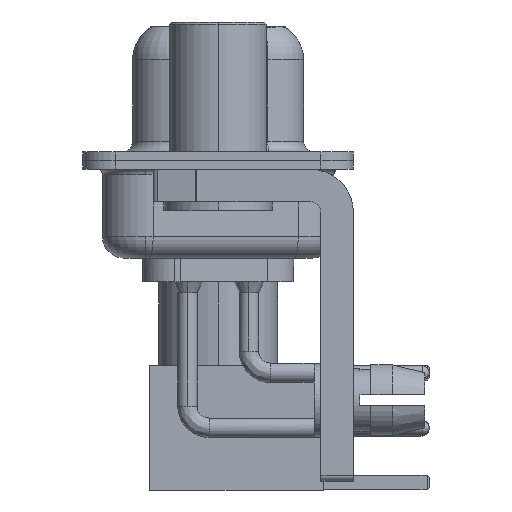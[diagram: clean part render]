
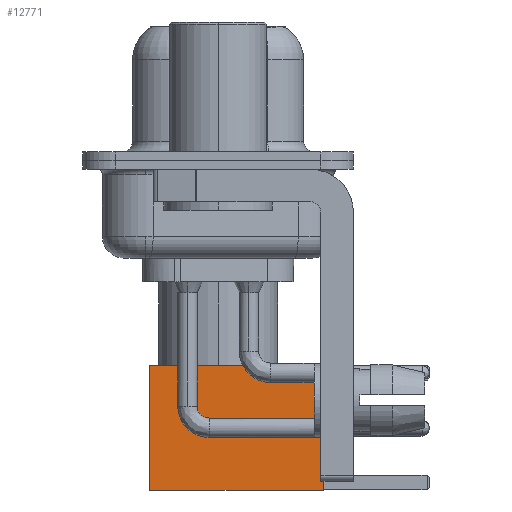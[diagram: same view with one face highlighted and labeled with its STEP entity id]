
A CAD part, left-side view. The second image highlights one B-rep face of the part: STEP entity #12771.
In plain terms, the highlighted face is planar.
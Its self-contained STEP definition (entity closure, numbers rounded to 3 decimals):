
#80 = FACE_OUTER_BOUND ( 'NONE', #11732, .T. ) ;
#1026 = LINE ( 'NONE', #19393, #6823 ) ;
#2244 = DIRECTION ( 'NONE',  ( 0., 0., -1. ) ) ;
#2800 = CARTESIAN_POINT ( 'NONE',  ( 2.875, 2.875, 8. ) ) ;
#3455 = ORIENTED_EDGE ( 'NONE', *, *, #25494, .T. ) ;
#4696 = DIRECTION ( 'NONE',  ( 0., 0., 1. ) ) ;
#6823 = VECTOR ( 'NONE', #12437, 1000. ) ;
#7174 = LINE ( 'NONE', #13538, #25326 ) ;
#7353 = CARTESIAN_POINT ( 'NONE',  ( 2.875, 2.875, 0. ) ) ;
#7496 = AXIS2_PLACEMENT_3D ( 'NONE', #7353, #24846, #4696 ) ;
#7610 = CARTESIAN_POINT ( 'NONE',  ( -2.875, 2.875, 0. ) ) ;
#9990 = VERTEX_POINT ( 'NONE', #13972 ) ;
#11001 = CARTESIAN_POINT ( 'NONE',  ( 0., 2.875, 0. ) ) ;
#11732 = EDGE_LOOP ( 'NONE', ( #18756, #3455, #27159, #20647 ) ) ;
#12437 = DIRECTION ( 'NONE',  ( -1., 0., 0. ) ) ;
#12771 = ADVANCED_FACE ( 'NONE', ( #80 ), #25289, .T. ) ;
#13538 = CARTESIAN_POINT ( 'NONE',  ( -2.875, 2.875, 0. ) ) ;
#13972 = CARTESIAN_POINT ( 'NONE',  ( -2.875, 2.875, 8. ) ) ;
#15745 = DIRECTION ( 'NONE',  ( 0., 0., -1. ) ) ;
#16915 = VECTOR ( 'NONE', #2244, 1000. ) ;
#18756 = ORIENTED_EDGE ( 'NONE', *, *, #24682, .T. ) ;
#19251 = EDGE_CURVE ( 'NONE', #28354, #9990, #1026, .T. ) ;
#19393 = CARTESIAN_POINT ( 'NONE',  ( 0., 2.875, 8. ) ) ;
#20495 = EDGE_CURVE ( 'NONE', #9990, #23976, #7174, .T. ) ;
#20647 = ORIENTED_EDGE ( 'NONE', *, *, #19251, .F. ) ;
#21230 = VECTOR ( 'NONE', #24486, 1000. ) ;
#23976 = VERTEX_POINT ( 'NONE', #7610 ) ;
#24486 = DIRECTION ( 'NONE',  ( -1., 0., 0. ) ) ;
#24682 = EDGE_CURVE ( 'NONE', #28354, #26234, #27287, .T. ) ;
#24846 = DIRECTION ( 'NONE',  ( 0., 1., 0. ) ) ;
#25289 = PLANE ( 'NONE',  #7496 ) ;
#25326 = VECTOR ( 'NONE', #15745, 1000. ) ;
#25494 = EDGE_CURVE ( 'NONE', #26234, #23976, #26713, .T. ) ;
#26234 = VERTEX_POINT ( 'NONE', #28150 ) ;
#26713 = LINE ( 'NONE', #11001, #21230 ) ;
#27159 = ORIENTED_EDGE ( 'NONE', *, *, #20495, .F. ) ;
#27287 = LINE ( 'NONE', #29226, #16915 ) ;
#28150 = CARTESIAN_POINT ( 'NONE',  ( 2.875, 2.875, 0. ) ) ;
#28354 = VERTEX_POINT ( 'NONE', #2800 ) ;
#29226 = CARTESIAN_POINT ( 'NONE',  ( 2.875, 2.875, 0. ) ) ;
